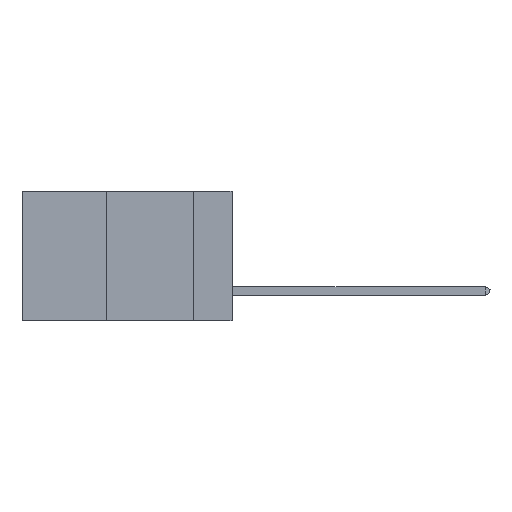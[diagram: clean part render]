
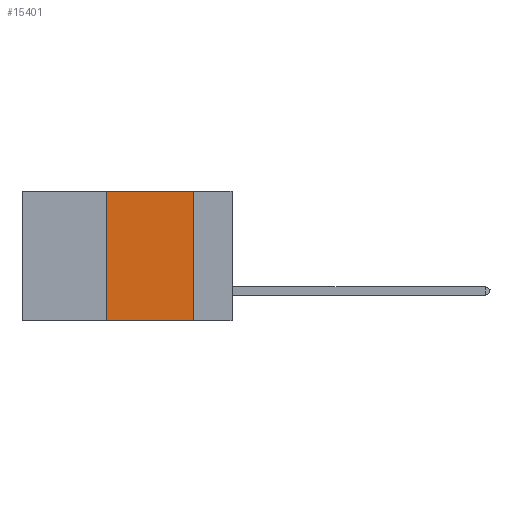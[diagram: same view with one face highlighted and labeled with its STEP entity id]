
A CAD part, left-side view. The second image highlights one B-rep face of the part: STEP entity #15401.
In plain terms, the highlighted planar face has unit normal (-1, 0, 0).
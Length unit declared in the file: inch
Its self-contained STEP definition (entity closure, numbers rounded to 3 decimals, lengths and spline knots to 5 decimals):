
#951 = ORIENTED_EDGE ( 'NONE', *, *, #8971, .F. ) ;
#1736 = DIRECTION ( 'NONE',  ( 0., 0., 1. ) ) ;
#2044 = CARTESIAN_POINT ( 'NONE',  ( 0., 0.36, 0. ) ) ;
#3679 = CARTESIAN_POINT ( 'NONE',  ( 0., 0.36, 0. ) ) ;
#4324 = ORIENTED_EDGE ( 'NONE', *, *, #19251, .F. ) ;
#4717 = DIRECTION ( 'NONE',  ( 0., 0., -1. ) ) ;
#5310 = ORIENTED_EDGE ( 'NONE', *, *, #7232, .T. ) ;
#5875 = VERTEX_POINT ( 'NONE', #6206 ) ;
#5975 = VERTEX_POINT ( 'NONE', #18679 ) ;
#6206 = CARTESIAN_POINT ( 'NONE',  ( 0., 0.36, -0.37 ) ) ;
#6325 = LINE ( 'NONE', #3679, #20455 ) ;
#6458 = DIRECTION ( 'NONE',  ( 1., 0., 0. ) ) ;
#7131 = CARTESIAN_POINT ( 'NONE',  ( 0., 0.6, 0. ) ) ;
#7232 = EDGE_CURVE ( 'NONE', #5875, #5975, #17727, .T. ) ;
#7287 = DIRECTION ( 'NONE',  ( 0., -1., 0. ) ) ;
#8467 = EDGE_CURVE ( 'NONE', #16586, #22673, #25829, .T. ) ;
#8971 = EDGE_CURVE ( 'NONE', #5875, #16586, #6325, .T. ) ;
#9251 = CARTESIAN_POINT ( 'NONE',  ( 0., 0.6, -0.37 ) ) ;
#9324 = DIRECTION ( 'NONE',  ( 0., -1., 0. ) ) ;
#9953 = CARTESIAN_POINT ( 'NONE',  ( 0., 0.11, 0. ) ) ;
#11882 = CARTESIAN_POINT ( 'NONE',  ( 0., 0.11, 0. ) ) ;
#11989 = DIRECTION ( 'NONE',  ( 0., 0., -1. ) ) ;
#12052 = VECTOR ( 'NONE', #9324, 39.37008 ) ;
#12533 = LINE ( 'NONE', #9953, #16943 ) ;
#13215 = FACE_OUTER_BOUND ( 'NONE', #16565, .T. ) ;
#15401 = ADVANCED_FACE ( 'NONE', ( #13215 ), #16577, .F. ) ;
#16565 = EDGE_LOOP ( 'NONE', ( #4324, #24415, #951, #5310 ) ) ;
#16577 = PLANE ( 'NONE',  #20032 ) ;
#16586 = VERTEX_POINT ( 'NONE', #2044 ) ;
#16943 = VECTOR ( 'NONE', #11989, 39.37008 ) ;
#17727 = LINE ( 'NONE', #9251, #19609 ) ;
#18679 = CARTESIAN_POINT ( 'NONE',  ( 0., 0.11, -0.37 ) ) ;
#19251 = EDGE_CURVE ( 'NONE', #22673, #5975, #12533, .T. ) ;
#19609 = VECTOR ( 'NONE', #7287, 39.37008 ) ;
#20032 = AXIS2_PLACEMENT_3D ( 'NONE', #20506, #6458, #4717 ) ;
#20455 = VECTOR ( 'NONE', #1736, 39.37008 ) ;
#20506 = CARTESIAN_POINT ( 'NONE',  ( 0., 0.6, 0. ) ) ;
#22673 = VERTEX_POINT ( 'NONE', #11882 ) ;
#24415 = ORIENTED_EDGE ( 'NONE', *, *, #8467, .F. ) ;
#25829 = LINE ( 'NONE', #7131, #12052 ) ;
